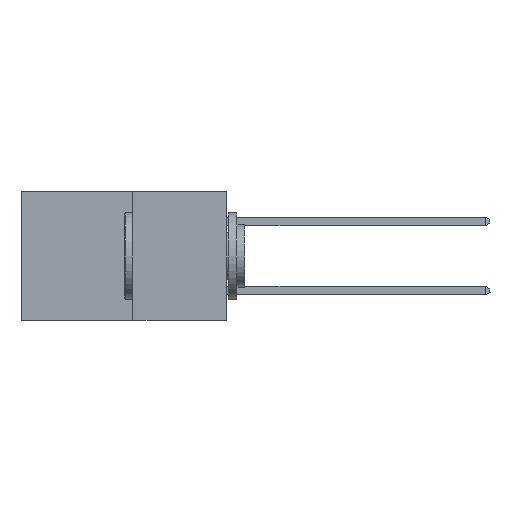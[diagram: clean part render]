
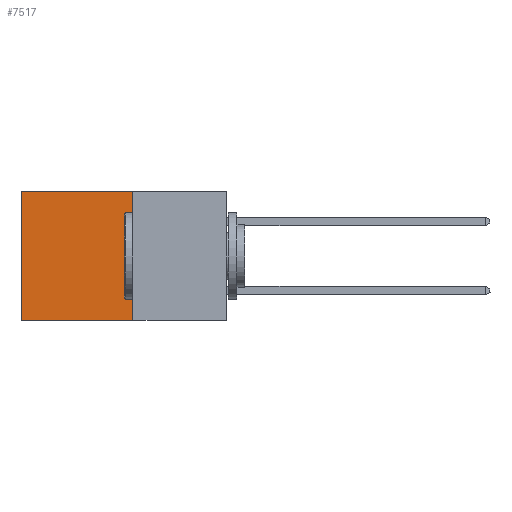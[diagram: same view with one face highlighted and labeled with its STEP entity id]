
A CAD part, left-side view. The second image highlights one B-rep face of the part: STEP entity #7517.
In plain terms, the highlighted planar face has unit normal (-1, 0, 0).
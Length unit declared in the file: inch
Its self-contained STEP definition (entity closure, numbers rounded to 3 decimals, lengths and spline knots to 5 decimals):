
#913 = EDGE_CURVE ( 'NONE', #20247, #13562, #17600, .T. ) ;
#3523 = ORIENTED_EDGE ( 'NONE', *, *, #21039, .F. ) ;
#3552 = VECTOR ( 'NONE', #14711, 39.37008 ) ;
#3558 = LINE ( 'NONE', #5751, #20497 ) ;
#4339 = CARTESIAN_POINT ( 'NONE',  ( 0.277, 0.59, 0. ) ) ;
#4716 = DIRECTION ( 'NONE',  ( 0., 0., -1. ) ) ;
#5751 = CARTESIAN_POINT ( 'NONE',  ( 0.277, 0.27, -0.37 ) ) ;
#6172 = LINE ( 'NONE', #6298, #14398 ) ;
#6298 = CARTESIAN_POINT ( 'NONE',  ( 0.277, 0.59, -0.37 ) ) ;
#7517 = ADVANCED_FACE ( 'NONE', ( #16322 ), #17181, .F. ) ;
#7599 = ORIENTED_EDGE ( 'NONE', *, *, #913, .T. ) ;
#7778 = VERTEX_POINT ( 'NONE', #11185 ) ;
#8525 = CARTESIAN_POINT ( 'NONE',  ( 0.277, 0.27, -0.37 ) ) ;
#8867 = VECTOR ( 'NONE', #11127, 39.37008 ) ;
#8989 = DIRECTION ( 'NONE',  ( 1., 0., 0. ) ) ;
#9103 = DIRECTION ( 'NONE',  ( 0., 0., -1. ) ) ;
#9499 = CARTESIAN_POINT ( 'NONE',  ( 0.277, 0.27, 0. ) ) ;
#9777 = AXIS2_PLACEMENT_3D ( 'NONE', #15532, #8989, #20471 ) ;
#10152 = VERTEX_POINT ( 'NONE', #8525 ) ;
#10948 = ORIENTED_EDGE ( 'NONE', *, *, #16193, .F. ) ;
#11127 = DIRECTION ( 'NONE',  ( 0., 1., 0. ) ) ;
#11185 = CARTESIAN_POINT ( 'NONE',  ( 0.277, 0.59, -0.37 ) ) ;
#11344 = ORIENTED_EDGE ( 'NONE', *, *, #14453, .T. ) ;
#12927 = CARTESIAN_POINT ( 'NONE',  ( 0.277, 0.27, 0. ) ) ;
#13562 = VERTEX_POINT ( 'NONE', #4339 ) ;
#14398 = VECTOR ( 'NONE', #4716, 39.37008 ) ;
#14453 = EDGE_CURVE ( 'NONE', #13562, #7778, #6172, .T. ) ;
#14711 = DIRECTION ( 'NONE',  ( 0., 1., 0. ) ) ;
#15532 = CARTESIAN_POINT ( 'NONE',  ( 0.277, 0.27, -0.37 ) ) ;
#15570 = EDGE_LOOP ( 'NONE', ( #11344, #3523, #10948, #7599 ) ) ;
#16193 = EDGE_CURVE ( 'NONE', #20247, #10152, #3558, .T. ) ;
#16322 = FACE_OUTER_BOUND ( 'NONE', #15570, .T. ) ;
#16646 = LINE ( 'NONE', #19658, #3552 ) ;
#17181 = PLANE ( 'NONE',  #9777 ) ;
#17600 = LINE ( 'NONE', #9499, #8867 ) ;
#19658 = CARTESIAN_POINT ( 'NONE',  ( 0.277, 0.27, -0.37 ) ) ;
#20247 = VERTEX_POINT ( 'NONE', #12927 ) ;
#20471 = DIRECTION ( 'NONE',  ( 0., 0., -1. ) ) ;
#20497 = VECTOR ( 'NONE', #9103, 39.37008 ) ;
#21039 = EDGE_CURVE ( 'NONE', #10152, #7778, #16646, .T. ) ;
